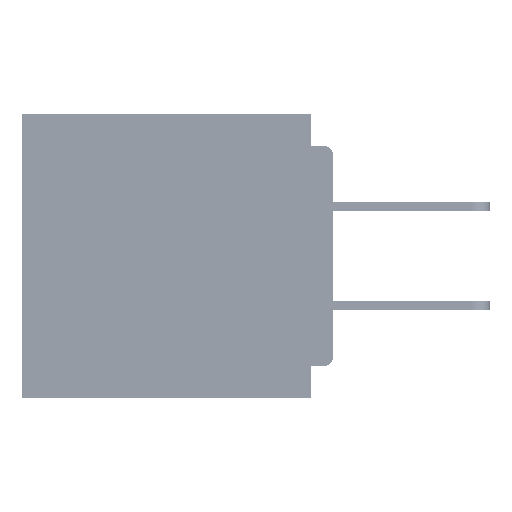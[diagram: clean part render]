
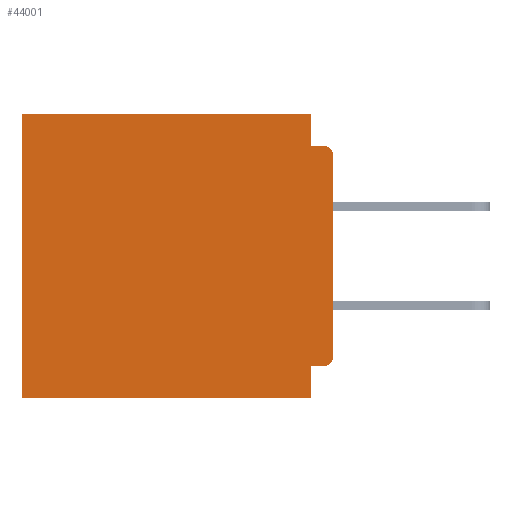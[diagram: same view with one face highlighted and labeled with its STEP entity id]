
A CAD part, left-side view. The second image highlights one B-rep face of the part: STEP entity #44001.
In plain terms, the highlighted planar face has unit normal (-1, 0, 0).
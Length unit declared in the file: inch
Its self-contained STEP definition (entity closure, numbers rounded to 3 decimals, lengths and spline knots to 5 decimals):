
#2529 = VERTEX_POINT ( 'NONE', #56491 ) ;
#4226 = EDGE_CURVE ( 'NONE', #32010, #2529, #57134, .T. ) ;
#4779 = DIRECTION ( 'NONE',  ( -1., 0., 0. ) ) ;
#5090 = DIRECTION ( 'NONE',  ( -1., 0., 0. ) ) ;
#6769 = AXIS2_PLACEMENT_3D ( 'NONE', #35704, #4779, #40871 ) ;
#7206 = CARTESIAN_POINT ( 'NONE',  ( 0.3, 0., -0.4 ) ) ;
#8462 = ORIENTED_EDGE ( 'NONE', *, *, #63050, .F. ) ;
#9145 = ORIENTED_EDGE ( 'NONE', *, *, #11793, .T. ) ;
#10372 = VERTEX_POINT ( 'NONE', #48468 ) ;
#11793 = EDGE_CURVE ( 'NONE', #25696, #2529, #60265, .T. ) ;
#11951 = CARTESIAN_POINT ( 'NONE',  ( 0.3, 0., -0.4 ) ) ;
#12743 = VECTOR ( 'NONE', #22564, 39.37008 ) ;
#16452 = ORIENTED_EDGE ( 'NONE', *, *, #22271, .T. ) ;
#17155 = DIRECTION ( 'NONE',  ( 1., 0., 0. ) ) ;
#17196 = LINE ( 'NONE', #42325, #43034 ) ;
#17830 = DIRECTION ( 'NONE',  ( 0., 0., -1. ) ) ;
#17974 = DIRECTION ( 'NONE',  ( 0., 0., -1. ) ) ;
#18049 = CARTESIAN_POINT ( 'NONE',  ( 0.3, 0., -0.06 ) ) ;
#18600 = VERTEX_POINT ( 'NONE', #18049 ) ;
#19180 = VECTOR ( 'NONE', #35036, 39.37008 ) ;
#19778 = ORIENTED_EDGE ( 'NONE', *, *, #32954, .F. ) ;
#19854 = VECTOR ( 'NONE', #47253, 39.37008 ) ;
#20779 = LINE ( 'NONE', #34806, #19180 ) ;
#21100 = EDGE_CURVE ( 'NONE', #35031, #49922, #50450, .T. ) ;
#22140 = LINE ( 'NONE', #43548, #47932 ) ;
#22271 = EDGE_CURVE ( 'NONE', #35031, #25696, #17196, .T. ) ;
#22564 = DIRECTION ( 'NONE',  ( 0., 1., 0. ) ) ;
#23706 = CARTESIAN_POINT ( 'NONE',  ( 0.3, 0.031, -0.4 ) ) ;
#23768 = DIRECTION ( 'NONE',  ( 0., 0., -1. ) ) ;
#25299 = ORIENTED_EDGE ( 'NONE', *, *, #41573, .T. ) ;
#25696 = VERTEX_POINT ( 'NONE', #60504 ) ;
#26797 = CARTESIAN_POINT ( 'NONE',  ( 0.3, 0., -0.045 ) ) ;
#26898 = AXIS2_PLACEMENT_3D ( 'NONE', #36006, #5090, #41178 ) ;
#28396 = CARTESIAN_POINT ( 'NONE',  ( 0.3, 0.031, 0. ) ) ;
#28606 = LINE ( 'NONE', #23706, #43892 ) ;
#28959 = CARTESIAN_POINT ( 'NONE',  ( 0.3, 0.437, -0.4 ) ) ;
#29832 = CIRCLE ( 'NONE', #26898, 0.015 ) ;
#30655 = VERTEX_POINT ( 'NONE', #58365 ) ;
#31930 = ORIENTED_EDGE ( 'NONE', *, *, #35773, .T. ) ;
#31947 = LINE ( 'NONE', #26797, #19854 ) ;
#32010 = VERTEX_POINT ( 'NONE', #49419 ) ;
#32583 = ORIENTED_EDGE ( 'NONE', *, *, #21100, .F. ) ;
#32954 = EDGE_CURVE ( 'NONE', #10372, #32010, #28606, .T. ) ;
#34806 = CARTESIAN_POINT ( 'NONE',  ( 0.3, 0., -0.355 ) ) ;
#34978 = CARTESIAN_POINT ( 'NONE',  ( 0.3, 0.015, -0.045 ) ) ;
#35031 = VERTEX_POINT ( 'NONE', #51164 ) ;
#35036 = DIRECTION ( 'NONE',  ( 0., 1., 0. ) ) ;
#35704 = CARTESIAN_POINT ( 'NONE',  ( 0.3, 0.015, -0.06 ) ) ;
#35773 = EDGE_CURVE ( 'NONE', #30655, #47141, #29832, .T. ) ;
#36006 = CARTESIAN_POINT ( 'NONE',  ( 0.3, 0.015, -0.34 ) ) ;
#40712 = FACE_OUTER_BOUND ( 'NONE', #54649, .T. ) ;
#40871 = DIRECTION ( 'NONE',  ( 0., 0., -1. ) ) ;
#41178 = DIRECTION ( 'NONE',  ( 0., 0., -1. ) ) ;
#41524 = ORIENTED_EDGE ( 'NONE', *, *, #4226, .F. ) ;
#41573 = EDGE_CURVE ( 'NONE', #18600, #42495, #43476, .T. ) ;
#42325 = CARTESIAN_POINT ( 'NONE',  ( 0.3, 0., 0. ) ) ;
#42495 = VERTEX_POINT ( 'NONE', #34978 ) ;
#42882 = PLANE ( 'NONE',  #62081 ) ;
#43034 = VECTOR ( 'NONE', #47483, 39.37008 ) ;
#43476 = CIRCLE ( 'NONE', #6769, 0.015 ) ;
#43548 = CARTESIAN_POINT ( 'NONE',  ( 0.3, 0., -0.4 ) ) ;
#43892 = VECTOR ( 'NONE', #49372, 39.37008 ) ;
#44001 = ADVANCED_FACE ( 'NONE', ( #40712 ), #42882, .F. ) ;
#44075 = EDGE_CURVE ( 'NONE', #18600, #47141, #22140, .T. ) ;
#44591 = ORIENTED_EDGE ( 'NONE', *, *, #44075, .F. ) ;
#46596 = VECTOR ( 'NONE', #23768, 39.37008 ) ;
#47141 = VERTEX_POINT ( 'NONE', #52449 ) ;
#47209 = VECTOR ( 'NONE', #17974, 39.37008 ) ;
#47253 = DIRECTION ( 'NONE',  ( 0., -1., 0. ) ) ;
#47483 = DIRECTION ( 'NONE',  ( 0., 1., 0. ) ) ;
#47932 = VECTOR ( 'NONE', #17830, 39.37008 ) ;
#48468 = CARTESIAN_POINT ( 'NONE',  ( 0.3, 0.031, -0.355 ) ) ;
#49372 = DIRECTION ( 'NONE',  ( 0., 0., -1. ) ) ;
#49419 = CARTESIAN_POINT ( 'NONE',  ( 0.3, 0.031, -0.4 ) ) ;
#49922 = VERTEX_POINT ( 'NONE', #55017 ) ;
#50450 = LINE ( 'NONE', #28396, #47209 ) ;
#50843 = EDGE_CURVE ( 'NONE', #49922, #42495, #31947, .T. ) ;
#51164 = CARTESIAN_POINT ( 'NONE',  ( 0.3, 0.031, 0. ) ) ;
#51908 = ORIENTED_EDGE ( 'NONE', *, *, #50843, .F. ) ;
#52449 = CARTESIAN_POINT ( 'NONE',  ( 0.3, 0., -0.34 ) ) ;
#53223 = DIRECTION ( 'NONE',  ( 0., 0., -1. ) ) ;
#54649 = EDGE_LOOP ( 'NONE', ( #44591, #25299, #51908, #32583, #16452, #9145, #41524, #19778, #8462, #31930 ) ) ;
#55017 = CARTESIAN_POINT ( 'NONE',  ( 0.3, 0.031, -0.045 ) ) ;
#56491 = CARTESIAN_POINT ( 'NONE',  ( 0.3, 0.437, -0.4 ) ) ;
#57134 = LINE ( 'NONE', #7206, #12743 ) ;
#58365 = CARTESIAN_POINT ( 'NONE',  ( 0.3, 0.015, -0.355 ) ) ;
#60265 = LINE ( 'NONE', #28959, #46596 ) ;
#60504 = CARTESIAN_POINT ( 'NONE',  ( 0.3, 0.437, 0. ) ) ;
#62081 = AXIS2_PLACEMENT_3D ( 'NONE', #11951, #17155, #53223 ) ;
#63050 = EDGE_CURVE ( 'NONE', #30655, #10372, #20779, .T. ) ;
